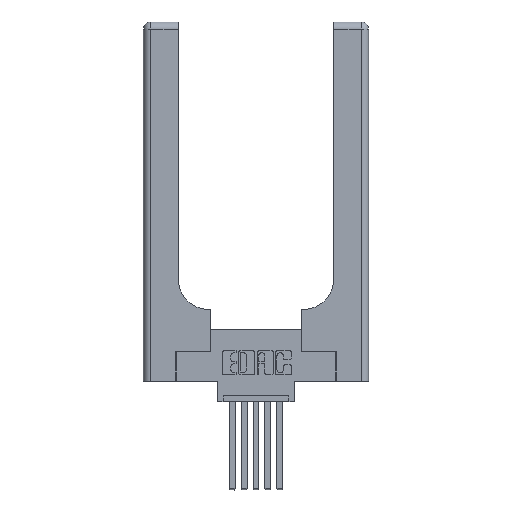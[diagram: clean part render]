
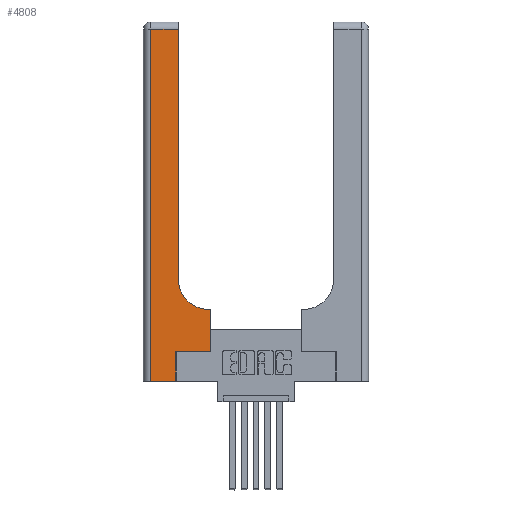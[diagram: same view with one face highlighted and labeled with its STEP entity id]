
A CAD part, top view. The second image highlights one B-rep face of the part: STEP entity #4808.
In plain terms, the highlighted planar face has unit normal (0, 0, 1).
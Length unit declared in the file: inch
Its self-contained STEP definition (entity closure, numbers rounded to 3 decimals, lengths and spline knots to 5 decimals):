
#507 = LINE ( 'NONE', #1677, #9551 ) ;
#673 = DIRECTION ( 'NONE',  ( 0., 0., -1. ) ) ;
#680 = CARTESIAN_POINT ( 'NONE',  ( 0.269, 0.25, 0.37 ) ) ;
#1007 = CARTESIAN_POINT ( 'NONE',  ( 0.2915, 0.6, 0.37 ) ) ;
#1068 = LINE ( 'NONE', #1538, #13826 ) ;
#1420 = VERTEX_POINT ( 'NONE', #7059 ) ;
#1495 = CARTESIAN_POINT ( 'NONE',  ( 0.5585, 0.6, 0.37 ) ) ;
#1538 = CARTESIAN_POINT ( 'NONE',  ( 0.2915, 3., 0.37 ) ) ;
#1677 = CARTESIAN_POINT ( 'NONE',  ( 0., 0., 0.37 ) ) ;
#1761 = ORIENTED_EDGE ( 'NONE', *, *, #7679, .T. ) ;
#1762 = DIRECTION ( 'NONE',  ( 0., -1., 0. ) ) ;
#1929 = VERTEX_POINT ( 'NONE', #7934 ) ;
#2531 = DIRECTION ( 'NONE',  ( 1., 0., 0. ) ) ;
#2684 = AXIS2_PLACEMENT_3D ( 'NONE', #6096, #673, #11447 ) ;
#2758 = CARTESIAN_POINT ( 'NONE',  ( 0.2915, 2.94, 0.37 ) ) ;
#2828 = LINE ( 'NONE', #3296, #10379 ) ;
#3296 = CARTESIAN_POINT ( 'NONE',  ( 0.269, 0., 0.37 ) ) ;
#3481 = VERTEX_POINT ( 'NONE', #13744 ) ;
#3650 = LINE ( 'NONE', #13257, #11362 ) ;
#3756 = DIRECTION ( 'NONE',  ( -1., 0., 0. ) ) ;
#3926 = CARTESIAN_POINT ( 'NONE',  ( 0.269, 0., 0.37 ) ) ;
#4680 = LINE ( 'NONE', #10205, #11216 ) ;
#4757 = ORIENTED_EDGE ( 'NONE', *, *, #10073, .T. ) ;
#4808 = ADVANCED_FACE ( 'NONE', ( #13447 ), #12481, .F. ) ;
#4862 = ORIENTED_EDGE ( 'NONE', *, *, #8110, .T. ) ;
#5005 = LINE ( 'NONE', #13506, #13903 ) ;
#5100 = DIRECTION ( 'NONE',  ( 1., 0., 0. ) ) ;
#5632 = ORIENTED_EDGE ( 'NONE', *, *, #13581, .T. ) ;
#5840 = CARTESIAN_POINT ( 'NONE',  ( 0.5415, 0.85, 0.37 ) ) ;
#6096 = CARTESIAN_POINT ( 'NONE',  ( 0., 3., 0.37 ) ) ;
#6153 = DIRECTION ( 'NONE',  ( 0., 1., 0. ) ) ;
#6342 = VERTEX_POINT ( 'NONE', #680 ) ;
#6346 = ORIENTED_EDGE ( 'NONE', *, *, #6911, .T. ) ;
#6840 = VECTOR ( 'NONE', #2531, 39.37008 ) ;
#6911 = EDGE_CURVE ( 'NONE', #3481, #11670, #507, .T. ) ;
#6997 = DIRECTION ( 'NONE',  ( 0., 0., -1. ) ) ;
#7059 = CARTESIAN_POINT ( 'NONE',  ( 0.5415, 0.6, 0.37 ) ) ;
#7219 = VERTEX_POINT ( 'NONE', #2758 ) ;
#7415 = ORIENTED_EDGE ( 'NONE', *, *, #10612, .T. ) ;
#7493 = DIRECTION ( 'NONE',  ( -1., 0., 0. ) ) ;
#7507 = EDGE_CURVE ( 'NONE', #13231, #3481, #5005, .T. ) ;
#7605 = EDGE_LOOP ( 'NONE', ( #5632, #9294, #7971, #6346, #1761, #4757, #4862, #7828, #7415 ) ) ;
#7646 = LINE ( 'NONE', #7938, #6840 ) ;
#7679 = EDGE_CURVE ( 'NONE', #11670, #6342, #2828, .T. ) ;
#7828 = ORIENTED_EDGE ( 'NONE', *, *, #10819, .T. ) ;
#7917 = DIRECTION ( 'NONE',  ( 1., 0., 0. ) ) ;
#7934 = CARTESIAN_POINT ( 'NONE',  ( 0.5585, 0.25, 0.37 ) ) ;
#7938 = CARTESIAN_POINT ( 'NONE',  ( 0.269, 0.25, 0.37 ) ) ;
#7971 = ORIENTED_EDGE ( 'NONE', *, *, #7507, .T. ) ;
#8110 = EDGE_CURVE ( 'NONE', #1929, #13610, #3650, .T. ) ;
#9020 = DIRECTION ( 'NONE',  ( 0., 1., 0. ) ) ;
#9043 = CARTESIAN_POINT ( 'NONE',  ( 0.2915, 0.85, 0.37 ) ) ;
#9294 = ORIENTED_EDGE ( 'NONE', *, *, #10283, .T. ) ;
#9520 = VECTOR ( 'NONE', #7493, 39.37008 ) ;
#9551 = VECTOR ( 'NONE', #5100, 39.37008 ) ;
#9756 = DIRECTION ( 'NONE',  ( 0., 1., 0. ) ) ;
#10073 = EDGE_CURVE ( 'NONE', #6342, #1929, #7646, .T. ) ;
#10137 = CARTESIAN_POINT ( 'NONE',  ( 0.06, 2.94, 0.37 ) ) ;
#10205 = CARTESIAN_POINT ( 'NONE',  ( 0., 2.94, 0.37 ) ) ;
#10283 = EDGE_CURVE ( 'NONE', #7219, #13231, #4680, .T. ) ;
#10374 = CIRCLE ( 'NONE', #12178, 0.25 ) ;
#10379 = VECTOR ( 'NONE', #9756, 39.37008 ) ;
#10612 = EDGE_CURVE ( 'NONE', #1420, #12755, #10374, .T. ) ;
#10819 = EDGE_CURVE ( 'NONE', #13610, #1420, #11369, .T. ) ;
#11216 = VECTOR ( 'NONE', #3756, 39.37008 ) ;
#11362 = VECTOR ( 'NONE', #6153, 39.37008 ) ;
#11369 = LINE ( 'NONE', #1007, #9520 ) ;
#11447 = DIRECTION ( 'NONE',  ( -1., 0., 0. ) ) ;
#11670 = VERTEX_POINT ( 'NONE', #3926 ) ;
#12178 = AXIS2_PLACEMENT_3D ( 'NONE', #5840, #6997, #7917 ) ;
#12481 = PLANE ( 'NONE',  #2684 ) ;
#12755 = VERTEX_POINT ( 'NONE', #9043 ) ;
#13231 = VERTEX_POINT ( 'NONE', #10137 ) ;
#13257 = CARTESIAN_POINT ( 'NONE',  ( 0.5585, 0.25, 0.37 ) ) ;
#13447 = FACE_OUTER_BOUND ( 'NONE', #7605, .T. ) ;
#13506 = CARTESIAN_POINT ( 'NONE',  ( 0.06, 3., 0.37 ) ) ;
#13581 = EDGE_CURVE ( 'NONE', #12755, #7219, #1068, .T. ) ;
#13610 = VERTEX_POINT ( 'NONE', #1495 ) ;
#13744 = CARTESIAN_POINT ( 'NONE',  ( 0.06, 0., 0.37 ) ) ;
#13826 = VECTOR ( 'NONE', #9020, 39.37008 ) ;
#13903 = VECTOR ( 'NONE', #1762, 39.37008 ) ;
